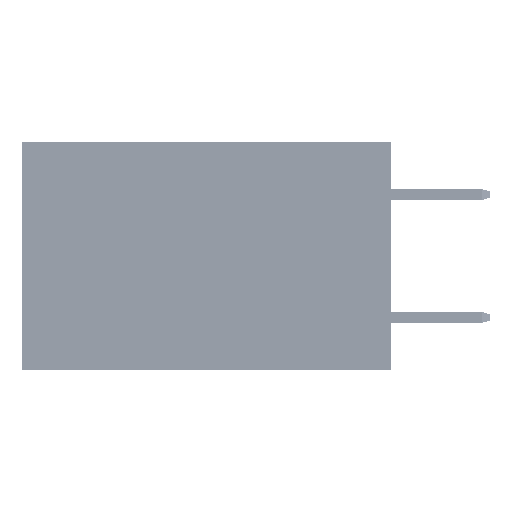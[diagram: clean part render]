
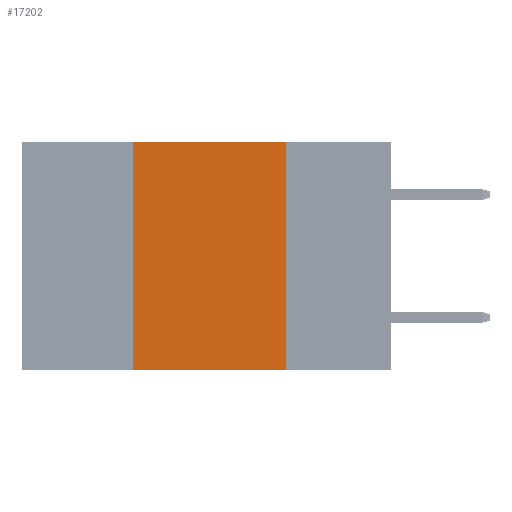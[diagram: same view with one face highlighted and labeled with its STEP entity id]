
A CAD part, left-side view. The second image highlights one B-rep face of the part: STEP entity #17202.
In plain terms, the highlighted planar face has unit normal (-1, 0, 0).
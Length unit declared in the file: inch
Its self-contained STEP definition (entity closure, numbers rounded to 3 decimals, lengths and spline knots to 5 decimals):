
#10 = CARTESIAN_POINT ( 'NONE',  ( 0., 0.6, -0.37 ) ) ;
#1894 = CARTESIAN_POINT ( 'NONE',  ( 0., 0.42, 0. ) ) ;
#2769 = EDGE_CURVE ( 'NONE', #41818, #32508, #21957, .T. ) ;
#3155 = VERTEX_POINT ( 'NONE', #1894 ) ;
#4667 = EDGE_LOOP ( 'NONE', ( #24208, #31636, #6046, #8730 ) ) ;
#6046 = ORIENTED_EDGE ( 'NONE', *, *, #35044, .F. ) ;
#7107 = EDGE_CURVE ( 'NONE', #3155, #8728, #23145, .T. ) ;
#7916 = DIRECTION ( 'NONE',  ( 0., -1., 0. ) ) ;
#8138 = LINE ( 'NONE', #43655, #27096 ) ;
#8728 = VERTEX_POINT ( 'NONE', #46029 ) ;
#8730 = ORIENTED_EDGE ( 'NONE', *, *, #2769, .T. ) ;
#12771 = VECTOR ( 'NONE', #7916, 39.37008 ) ;
#15654 = FACE_OUTER_BOUND ( 'NONE', #4667, .T. ) ;
#16349 = VECTOR ( 'NONE', #49376, 39.37008 ) ;
#17202 = ADVANCED_FACE ( 'NONE', ( #15654 ), #35432, .F. ) ;
#20046 = CARTESIAN_POINT ( 'NONE',  ( 0., 0.6, 0. ) ) ;
#21701 = AXIS2_PLACEMENT_3D ( 'NONE', #20046, #31376, #27781 ) ;
#21957 = LINE ( 'NONE', #10, #37253 ) ;
#23145 = LINE ( 'NONE', #46928, #12771 ) ;
#24208 = ORIENTED_EDGE ( 'NONE', *, *, #49872, .F. ) ;
#27096 = VECTOR ( 'NONE', #47765, 39.37008 ) ;
#27437 = DIRECTION ( 'NONE',  ( 0., -1., 0. ) ) ;
#27781 = DIRECTION ( 'NONE',  ( 0., 0., -1. ) ) ;
#30468 = CARTESIAN_POINT ( 'NONE',  ( 0., 0.42, -0.37 ) ) ;
#31376 = DIRECTION ( 'NONE',  ( 1., 0., 0. ) ) ;
#31636 = ORIENTED_EDGE ( 'NONE', *, *, #7107, .F. ) ;
#32508 = VERTEX_POINT ( 'NONE', #32831 ) ;
#32831 = CARTESIAN_POINT ( 'NONE',  ( 0., 0.17, -0.37 ) ) ;
#33575 = CARTESIAN_POINT ( 'NONE',  ( 0., 0.42, 0. ) ) ;
#35044 = EDGE_CURVE ( 'NONE', #41818, #3155, #48888, .T. ) ;
#35432 = PLANE ( 'NONE',  #21701 ) ;
#37253 = VECTOR ( 'NONE', #27437, 39.37008 ) ;
#41818 = VERTEX_POINT ( 'NONE', #30468 ) ;
#43655 = CARTESIAN_POINT ( 'NONE',  ( 0., 0.17, 0. ) ) ;
#46029 = CARTESIAN_POINT ( 'NONE',  ( 0., 0.17, 0. ) ) ;
#46928 = CARTESIAN_POINT ( 'NONE',  ( 0., 0.6, 0. ) ) ;
#47765 = DIRECTION ( 'NONE',  ( 0., 0., -1. ) ) ;
#48888 = LINE ( 'NONE', #33575, #16349 ) ;
#49376 = DIRECTION ( 'NONE',  ( 0., 0., 1. ) ) ;
#49872 = EDGE_CURVE ( 'NONE', #8728, #32508, #8138, .T. ) ;
